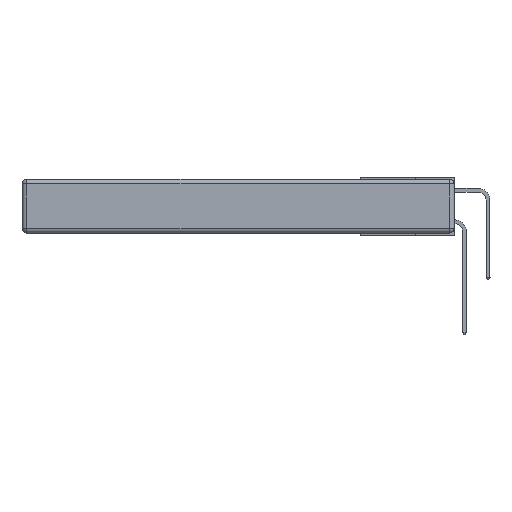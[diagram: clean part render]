
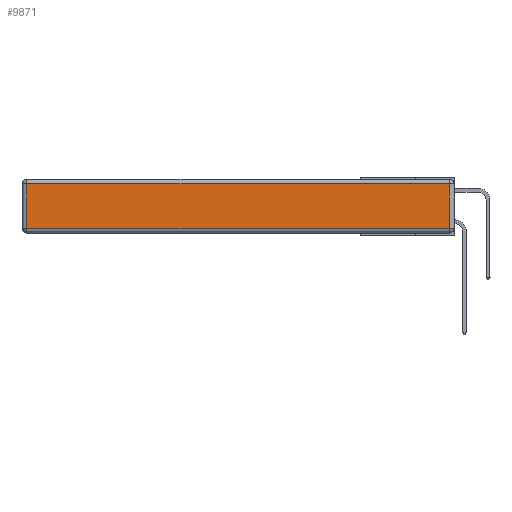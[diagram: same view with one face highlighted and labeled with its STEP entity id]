
A CAD part, left-side view. The second image highlights one B-rep face of the part: STEP entity #9871.
In plain terms, the highlighted planar face has unit normal (-1, 0, 0).
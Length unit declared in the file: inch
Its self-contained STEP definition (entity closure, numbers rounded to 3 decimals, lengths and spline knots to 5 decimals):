
#240 = CARTESIAN_POINT ( 'NONE',  ( 0., 0.03, -0.03 ) ) ;
#705 = ORIENTED_EDGE ( 'NONE', *, *, #6051, .T. ) ;
#925 = LINE ( 'NONE', #19525, #5533 ) ;
#949 = DIRECTION ( 'NONE',  ( -1., 0., 0. ) ) ;
#1848 = DIRECTION ( 'NONE',  ( 0., 0., 1. ) ) ;
#2120 = VECTOR ( 'NONE', #25133, 39.37008 ) ;
#5290 = ORIENTED_EDGE ( 'NONE', *, *, #7331, .T. ) ;
#5533 = VECTOR ( 'NONE', #1848, 39.37008 ) ;
#6051 = EDGE_CURVE ( 'NONE', #15674, #6526, #23521, .T. ) ;
#6073 = CARTESIAN_POINT ( 'NONE',  ( 0., 2.75, -0.03 ) ) ;
#6526 = VERTEX_POINT ( 'NONE', #12915 ) ;
#6969 = ORIENTED_EDGE ( 'NONE', *, *, #18778, .T. ) ;
#6976 = CARTESIAN_POINT ( 'NONE',  ( 0., 0., -0.343 ) ) ;
#7331 = EDGE_CURVE ( 'NONE', #16550, #15674, #925, .T. ) ;
#7341 = LINE ( 'NONE', #9153, #2120 ) ;
#7928 = AXIS2_PLACEMENT_3D ( 'NONE', #6976, #949, #18794 ) ;
#9153 = CARTESIAN_POINT ( 'NONE',  ( 0., 0., -0.313 ) ) ;
#9871 = ADVANCED_FACE ( 'NONE', ( #17711 ), #16892, .T. ) ;
#10841 = VECTOR ( 'NONE', #12010, 39.37008 ) ;
#11343 = DIRECTION ( 'NONE',  ( 0., 0., -1. ) ) ;
#12010 = DIRECTION ( 'NONE',  ( 0., 1., 0. ) ) ;
#12487 = EDGE_LOOP ( 'NONE', ( #6969, #5290, #705, #23480 ) ) ;
#12915 = CARTESIAN_POINT ( 'NONE',  ( 0., 2.72, -0.03 ) ) ;
#14859 = CARTESIAN_POINT ( 'NONE',  ( 0., 0.03, -0.313 ) ) ;
#14940 = VECTOR ( 'NONE', #11343, 39.37008 ) ;
#15319 = VERTEX_POINT ( 'NONE', #16246 ) ;
#15674 = VERTEX_POINT ( 'NONE', #240 ) ;
#15793 = EDGE_CURVE ( 'NONE', #6526, #15319, #16499, .T. ) ;
#16246 = CARTESIAN_POINT ( 'NONE',  ( 0., 2.72, -0.313 ) ) ;
#16499 = LINE ( 'NONE', #23197, #14940 ) ;
#16550 = VERTEX_POINT ( 'NONE', #14859 ) ;
#16892 = PLANE ( 'NONE',  #7928 ) ;
#17711 = FACE_OUTER_BOUND ( 'NONE', #12487, .T. ) ;
#18778 = EDGE_CURVE ( 'NONE', #15319, #16550, #7341, .T. ) ;
#18794 = DIRECTION ( 'NONE',  ( 0., 0., 1. ) ) ;
#19525 = CARTESIAN_POINT ( 'NONE',  ( 0., 0.03, -0.343 ) ) ;
#23197 = CARTESIAN_POINT ( 'NONE',  ( 0., 2.72, -0.343 ) ) ;
#23480 = ORIENTED_EDGE ( 'NONE', *, *, #15793, .T. ) ;
#23521 = LINE ( 'NONE', #6073, #10841 ) ;
#25133 = DIRECTION ( 'NONE',  ( 0., -1., 0. ) ) ;
